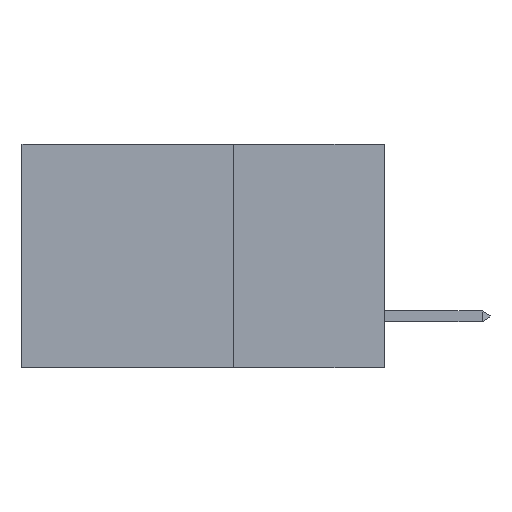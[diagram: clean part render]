
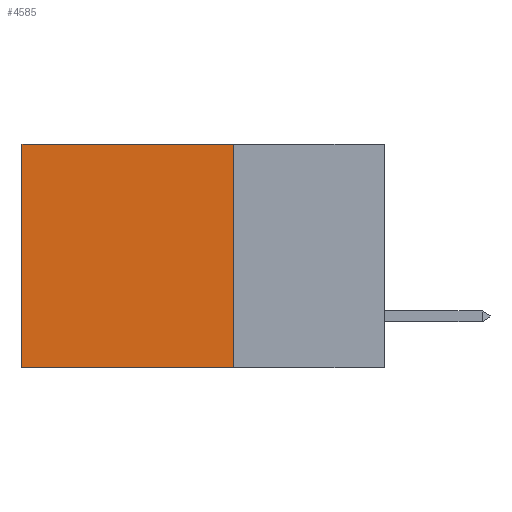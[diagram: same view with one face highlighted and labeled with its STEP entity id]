
A CAD part, left-side view. The second image highlights one B-rep face of the part: STEP entity #4585.
In plain terms, the highlighted planar face has unit normal (-1, 0, 0).
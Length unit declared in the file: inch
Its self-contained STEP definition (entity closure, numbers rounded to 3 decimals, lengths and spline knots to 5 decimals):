
#428 = VECTOR ( 'NONE', #23327, 39.37008 ) ;
#1013 = CARTESIAN_POINT ( 'NONE',  ( 0.2875, 0.25, 0. ) ) ;
#3125 = LINE ( 'NONE', #5730, #428 ) ;
#3862 = CARTESIAN_POINT ( 'NONE',  ( 0.2875, 0.25, 0. ) ) ;
#4585 = ADVANCED_FACE ( 'NONE', ( #25754 ), #23323, .F. ) ;
#5730 = CARTESIAN_POINT ( 'NONE',  ( 0.2875, 0.25, -0.37 ) ) ;
#6226 = DIRECTION ( 'NONE',  ( 0., 0., -1. ) ) ;
#8140 = LINE ( 'NONE', #22485, #29377 ) ;
#9568 = VERTEX_POINT ( 'NONE', #18717 ) ;
#10089 = VECTOR ( 'NONE', #24201, 39.37008 ) ;
#11947 = EDGE_CURVE ( 'NONE', #30957, #9568, #8140, .T. ) ;
#13008 = ORIENTED_EDGE ( 'NONE', *, *, #25403, .T. ) ;
#14194 = ORIENTED_EDGE ( 'NONE', *, *, #19450, .F. ) ;
#14459 = VECTOR ( 'NONE', #21240, 39.37008 ) ;
#18604 = DIRECTION ( 'NONE',  ( 1., 0., 0. ) ) ;
#18717 = CARTESIAN_POINT ( 'NONE',  ( 0.2875, 0.6, 0. ) ) ;
#19119 = LINE ( 'NONE', #28558, #14459 ) ;
#19450 = EDGE_CURVE ( 'NONE', #30957, #31193, #23732, .T. ) ;
#19790 = CARTESIAN_POINT ( 'NONE',  ( 0.2875, 0.6, -0.37 ) ) ;
#20202 = DIRECTION ( 'NONE',  ( 0., 1., 0. ) ) ;
#21240 = DIRECTION ( 'NONE',  ( 0., 0., -1. ) ) ;
#22485 = CARTESIAN_POINT ( 'NONE',  ( 0.2875, 0.25, 0. ) ) ;
#22869 = ORIENTED_EDGE ( 'NONE', *, *, #30452, .F. ) ;
#23323 = PLANE ( 'NONE',  #23963 ) ;
#23327 = DIRECTION ( 'NONE',  ( 0., 1., 0. ) ) ;
#23732 = LINE ( 'NONE', #29085, #10089 ) ;
#23963 = AXIS2_PLACEMENT_3D ( 'NONE', #1013, #18604, #6226 ) ;
#24201 = DIRECTION ( 'NONE',  ( 0., 0., -1. ) ) ;
#25403 = EDGE_CURVE ( 'NONE', #9568, #29883, #19119, .T. ) ;
#25754 = FACE_OUTER_BOUND ( 'NONE', #31604, .T. ) ;
#28031 = ORIENTED_EDGE ( 'NONE', *, *, #11947, .T. ) ;
#28558 = CARTESIAN_POINT ( 'NONE',  ( 0.2875, 0.6, 0. ) ) ;
#28759 = CARTESIAN_POINT ( 'NONE',  ( 0.2875, 0.25, -0.37 ) ) ;
#29085 = CARTESIAN_POINT ( 'NONE',  ( 0.2875, 0.25, 0. ) ) ;
#29377 = VECTOR ( 'NONE', #20202, 39.37008 ) ;
#29883 = VERTEX_POINT ( 'NONE', #19790 ) ;
#30452 = EDGE_CURVE ( 'NONE', #31193, #29883, #3125, .T. ) ;
#30957 = VERTEX_POINT ( 'NONE', #3862 ) ;
#31193 = VERTEX_POINT ( 'NONE', #28759 ) ;
#31604 = EDGE_LOOP ( 'NONE', ( #13008, #22869, #14194, #28031 ) ) ;
